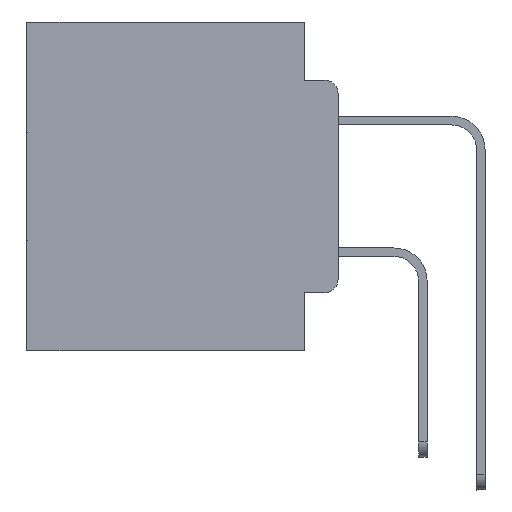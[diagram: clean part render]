
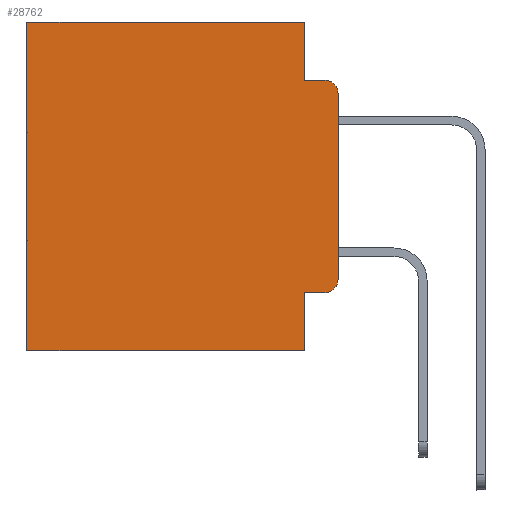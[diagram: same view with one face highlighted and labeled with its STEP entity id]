
A CAD part, left-side view. The second image highlights one B-rep face of the part: STEP entity #28762.
In plain terms, the highlighted planar face has unit normal (-1, 0, 0).
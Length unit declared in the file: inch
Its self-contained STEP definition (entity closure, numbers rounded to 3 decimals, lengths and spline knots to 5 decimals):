
#11 = VERTEX_POINT ( 'NONE', #12393 ) ;
#178 = PLANE ( 'NONE',  #16683 ) ;
#468 = VECTOR ( 'NONE', #3010, 39.37008 ) ;
#1807 = DIRECTION ( 'NONE',  ( 0., 1., 0. ) ) ;
#1890 = VECTOR ( 'NONE', #19549, 39.37008 ) ;
#2295 = CARTESIAN_POINT ( 'NONE',  ( 0.298, 0.02, -0.3915 ) ) ;
#2634 = EDGE_CURVE ( 'NONE', #22310, #19927, #22744, .T. ) ;
#2746 = DIRECTION ( 'NONE',  ( 1., 0., 0. ) ) ;
#2974 = EDGE_LOOP ( 'NONE', ( #12862, #24874, #8696, #11381, #23401, #9857, #21192, #28941, #3829, #23081 ) ) ;
#3010 = DIRECTION ( 'NONE',  ( 0., 0., -1. ) ) ;
#3143 = CARTESIAN_POINT ( 'NONE',  ( 0.298, 0.051, -0.4115 ) ) ;
#3677 = LINE ( 'NONE', #11582, #15846 ) ;
#3829 = ORIENTED_EDGE ( 'NONE', *, *, #21336, .T. ) ;
#4163 = VECTOR ( 'NONE', #6947, 39.37008 ) ;
#4622 = LINE ( 'NONE', #3143, #28656 ) ;
#4803 = DIRECTION ( 'NONE',  ( 0., 0., -1. ) ) ;
#5042 = EDGE_CURVE ( 'NONE', #22227, #25148, #3677, .T. ) ;
#6771 = VERTEX_POINT ( 'NONE', #27380 ) ;
#6947 = DIRECTION ( 'NONE',  ( 0., 0., -1. ) ) ;
#7323 = CARTESIAN_POINT ( 'NONE',  ( 0.298, 0.051, 0. ) ) ;
#7586 = CARTESIAN_POINT ( 'NONE',  ( 0.298, 0., 0. ) ) ;
#7827 = EDGE_CURVE ( 'NONE', #13102, #30680, #15344, .T. ) ;
#8510 = AXIS2_PLACEMENT_3D ( 'NONE', #25841, #11507, #28215 ) ;
#8618 = CARTESIAN_POINT ( 'NONE',  ( 0.298, 0.473, -0.5 ) ) ;
#8696 = ORIENTED_EDGE ( 'NONE', *, *, #2634, .F. ) ;
#9125 = DIRECTION ( 'NONE',  ( 0., 0., -1. ) ) ;
#9159 = VECTOR ( 'NONE', #9577, 39.37008 ) ;
#9350 = CARTESIAN_POINT ( 'NONE',  ( 0.298, 0.473, 0. ) ) ;
#9535 = CARTESIAN_POINT ( 'NONE',  ( 0.298, 0.02, -0.0885 ) ) ;
#9577 = DIRECTION ( 'NONE',  ( 0., -1., 0. ) ) ;
#9857 = ORIENTED_EDGE ( 'NONE', *, *, #22324, .T. ) ;
#9969 = LINE ( 'NONE', #17119, #1890 ) ;
#10058 = VERTEX_POINT ( 'NONE', #20017 ) ;
#10639 = LINE ( 'NONE', #9350, #4163 ) ;
#11381 = ORIENTED_EDGE ( 'NONE', *, *, #21142, .F. ) ;
#11387 = CARTESIAN_POINT ( 'NONE',  ( 0.298, 0., -0.1085 ) ) ;
#11507 = DIRECTION ( 'NONE',  ( -1., 0., 0. ) ) ;
#11582 = CARTESIAN_POINT ( 'NONE',  ( 0.298, 0., 0. ) ) ;
#12393 = CARTESIAN_POINT ( 'NONE',  ( 0.298, 0.473, 0. ) ) ;
#12862 = ORIENTED_EDGE ( 'NONE', *, *, #5042, .F. ) ;
#13102 = VERTEX_POINT ( 'NONE', #17056 ) ;
#13234 = EDGE_CURVE ( 'NONE', #6771, #13102, #30982, .T. ) ;
#13795 = CARTESIAN_POINT ( 'NONE',  ( 0.298, 0.051, -0.0885 ) ) ;
#14993 = LINE ( 'NONE', #30588, #22123 ) ;
#15138 = CARTESIAN_POINT ( 'NONE',  ( 0.298, 0.051, 0. ) ) ;
#15344 = LINE ( 'NONE', #19568, #27273 ) ;
#15846 = VECTOR ( 'NONE', #9125, 39.37008 ) ;
#16114 = CARTESIAN_POINT ( 'NONE',  ( 0.298, 0., -0.3915 ) ) ;
#16589 = CARTESIAN_POINT ( 'NONE',  ( 0.298, 0.051, -0.0885 ) ) ;
#16683 = AXIS2_PLACEMENT_3D ( 'NONE', #7586, #2746, #19769 ) ;
#17056 = CARTESIAN_POINT ( 'NONE',  ( 0.298, 0.051, -0.5 ) ) ;
#17119 = CARTESIAN_POINT ( 'NONE',  ( 0.298, 0.051, 0. ) ) ;
#17139 = DIRECTION ( 'NONE',  ( 0., 1., 0. ) ) ;
#19140 = EDGE_CURVE ( 'NONE', #22227, #19927, #23263, .T. ) ;
#19343 = DIRECTION ( 'NONE',  ( -1., 0., 0. ) ) ;
#19549 = DIRECTION ( 'NONE',  ( 0., 0., -1. ) ) ;
#19568 = CARTESIAN_POINT ( 'NONE',  ( 0.298, 0., -0.5 ) ) ;
#19769 = DIRECTION ( 'NONE',  ( 0., 0., -1. ) ) ;
#19807 = EDGE_CURVE ( 'NONE', #19947, #11, #14993, .T. ) ;
#19927 = VERTEX_POINT ( 'NONE', #9535 ) ;
#19947 = VERTEX_POINT ( 'NONE', #7323 ) ;
#20017 = CARTESIAN_POINT ( 'NONE',  ( 0.298, 0.02, -0.4115 ) ) ;
#21063 = EDGE_CURVE ( 'NONE', #10058, #25148, #29778, .T. ) ;
#21142 = EDGE_CURVE ( 'NONE', #19947, #22310, #9969, .T. ) ;
#21192 = ORIENTED_EDGE ( 'NONE', *, *, #7827, .F. ) ;
#21336 = EDGE_CURVE ( 'NONE', #6771, #10058, #4622, .T. ) ;
#21907 = FACE_OUTER_BOUND ( 'NONE', #2974, .T. ) ;
#22123 = VECTOR ( 'NONE', #1807, 39.37008 ) ;
#22227 = VERTEX_POINT ( 'NONE', #11387 ) ;
#22310 = VERTEX_POINT ( 'NONE', #16589 ) ;
#22324 = EDGE_CURVE ( 'NONE', #11, #30680, #10639, .T. ) ;
#22744 = LINE ( 'NONE', #13795, #9159 ) ;
#23081 = ORIENTED_EDGE ( 'NONE', *, *, #21063, .T. ) ;
#23263 = CIRCLE ( 'NONE', #8510, 0.02 ) ;
#23401 = ORIENTED_EDGE ( 'NONE', *, *, #19807, .T. ) ;
#24874 = ORIENTED_EDGE ( 'NONE', *, *, #19140, .T. ) ;
#25148 = VERTEX_POINT ( 'NONE', #16114 ) ;
#25841 = CARTESIAN_POINT ( 'NONE',  ( 0.298, 0.02, -0.1085 ) ) ;
#27273 = VECTOR ( 'NONE', #17139, 39.37008 ) ;
#27380 = CARTESIAN_POINT ( 'NONE',  ( 0.298, 0.051, -0.4115 ) ) ;
#27460 = AXIS2_PLACEMENT_3D ( 'NONE', #2295, #19343, #4803 ) ;
#28215 = DIRECTION ( 'NONE',  ( 0., 0., -1. ) ) ;
#28656 = VECTOR ( 'NONE', #29598, 39.37008 ) ;
#28762 = ADVANCED_FACE ( 'NONE', ( #21907 ), #178, .F. ) ;
#28941 = ORIENTED_EDGE ( 'NONE', *, *, #13234, .F. ) ;
#29598 = DIRECTION ( 'NONE',  ( 0., -1., 0. ) ) ;
#29778 = CIRCLE ( 'NONE', #27460, 0.02 ) ;
#30588 = CARTESIAN_POINT ( 'NONE',  ( 0.298, 0., 0. ) ) ;
#30680 = VERTEX_POINT ( 'NONE', #8618 ) ;
#30982 = LINE ( 'NONE', #15138, #468 ) ;
